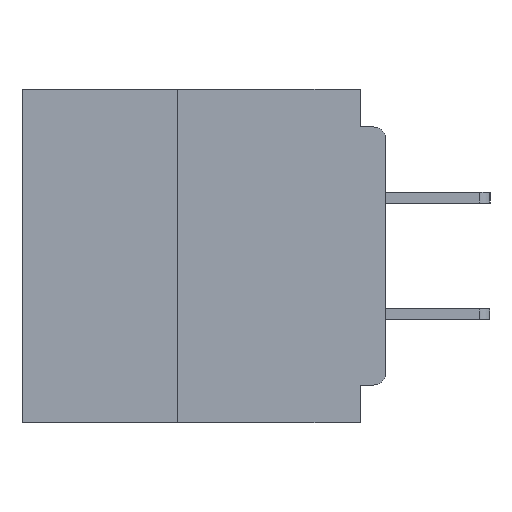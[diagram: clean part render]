
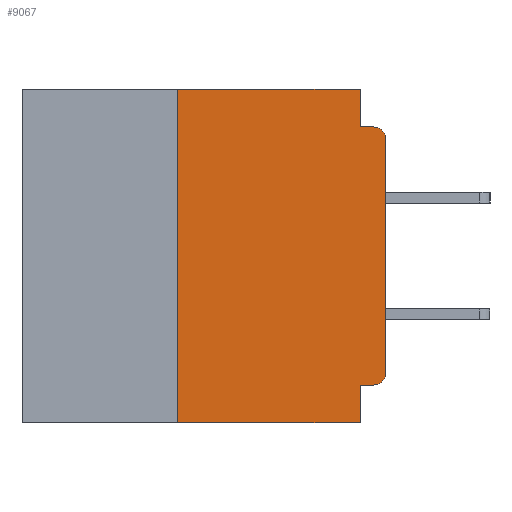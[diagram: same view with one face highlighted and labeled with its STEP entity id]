
A CAD part, left-side view. The second image highlights one B-rep face of the part: STEP entity #9067.
In plain terms, the highlighted planar face has unit normal (-1, 0, 0).
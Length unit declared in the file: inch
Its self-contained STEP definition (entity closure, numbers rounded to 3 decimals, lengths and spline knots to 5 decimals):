
#105 = CIRCLE ( 'NONE', #36105, 0.015 ) ;
#125 = ORIENTED_EDGE ( 'NONE', *, *, #11228, .F. ) ;
#563 = ORIENTED_EDGE ( 'NONE', *, *, #21620, .F. ) ;
#750 = DIRECTION ( 'NONE',  ( 0., 0., 1. ) ) ;
#1239 = CARTESIAN_POINT ( 'NONE',  ( 0., 0.031, -0.4 ) ) ;
#1869 = DIRECTION ( 'NONE',  ( 0., 1., 0. ) ) ;
#3515 = DIRECTION ( 'NONE',  ( 0., 0., -1. ) ) ;
#4103 = EDGE_LOOP ( 'NONE', ( #13863, #13553, #14789, #563, #125, #31696, #28280, #12062, #9687, #27639 ) ) ;
#4667 = CARTESIAN_POINT ( 'NONE',  ( 0., 0.031, 0. ) ) ;
#5023 = EDGE_CURVE ( 'NONE', #28924, #10430, #46100, .T. ) ;
#5041 = VERTEX_POINT ( 'NONE', #47145 ) ;
#5115 = CARTESIAN_POINT ( 'NONE',  ( 0., 0., -0.045 ) ) ;
#5302 = CARTESIAN_POINT ( 'NONE',  ( 0., 0.031, 0. ) ) ;
#5616 = LINE ( 'NONE', #36200, #42425 ) ;
#5753 = PLANE ( 'NONE',  #44428 ) ;
#6088 = VERTEX_POINT ( 'NONE', #42283 ) ;
#6740 = VECTOR ( 'NONE', #1869, 39.37008 ) ;
#6864 = EDGE_CURVE ( 'NONE', #41662, #24898, #14337, .T. ) ;
#8926 = EDGE_CURVE ( 'NONE', #46734, #6088, #25971, .T. ) ;
#9067 = ADVANCED_FACE ( 'NONE', ( #39708 ), #5753, .F. ) ;
#9687 = ORIENTED_EDGE ( 'NONE', *, *, #43727, .F. ) ;
#9796 = DIRECTION ( 'NONE',  ( -1., 0., 0. ) ) ;
#10430 = VERTEX_POINT ( 'NONE', #42661 ) ;
#10897 = CIRCLE ( 'NONE', #10925, 0.015 ) ;
#10925 = AXIS2_PLACEMENT_3D ( 'NONE', #47490, #25599, #3515 ) ;
#11228 = EDGE_CURVE ( 'NONE', #24898, #43051, #5616, .T. ) ;
#12062 = ORIENTED_EDGE ( 'NONE', *, *, #5023, .F. ) ;
#12547 = DIRECTION ( 'NONE',  ( 0., -1., 0. ) ) ;
#13178 = CARTESIAN_POINT ( 'NONE',  ( 0., 0.437, 0. ) ) ;
#13553 = ORIENTED_EDGE ( 'NONE', *, *, #17306, .T. ) ;
#13863 = ORIENTED_EDGE ( 'NONE', *, *, #33648, .T. ) ;
#14337 = LINE ( 'NONE', #16365, #32766 ) ;
#14789 = ORIENTED_EDGE ( 'NONE', *, *, #8926, .F. ) ;
#16158 = VECTOR ( 'NONE', #12547, 39.37008 ) ;
#16365 = CARTESIAN_POINT ( 'NONE',  ( 0., 0.25, -0.4 ) ) ;
#16842 = VECTOR ( 'NONE', #39131, 39.37008 ) ;
#17051 = DIRECTION ( 'NONE',  ( 0., 0., 1. ) ) ;
#17306 = EDGE_CURVE ( 'NONE', #38258, #6088, #105, .T. ) ;
#17694 = LINE ( 'NONE', #27653, #6740 ) ;
#17838 = DIRECTION ( 'NONE',  ( 0., -1., 0. ) ) ;
#20596 = DIRECTION ( 'NONE',  ( 1., 0., 0. ) ) ;
#21620 = EDGE_CURVE ( 'NONE', #43051, #46734, #24246, .T. ) ;
#21871 = LINE ( 'NONE', #43495, #41409 ) ;
#22121 = LINE ( 'NONE', #30200, #40483 ) ;
#22602 = CARTESIAN_POINT ( 'NONE',  ( 0., 0.25, -0.4 ) ) ;
#22712 = CARTESIAN_POINT ( 'NONE',  ( 0., 0.25, 0. ) ) ;
#24246 = LINE ( 'NONE', #4667, #32825 ) ;
#24295 = CARTESIAN_POINT ( 'NONE',  ( 0., 0.031, -0.045 ) ) ;
#24898 = VERTEX_POINT ( 'NONE', #22712 ) ;
#25599 = DIRECTION ( 'NONE',  ( -1., 0., 0. ) ) ;
#25788 = CARTESIAN_POINT ( 'NONE',  ( 0., 0.015, -0.355 ) ) ;
#25971 = LINE ( 'NONE', #5115, #16158 ) ;
#26922 = DIRECTION ( 'NONE',  ( 0., 0., -1. ) ) ;
#27639 = ORIENTED_EDGE ( 'NONE', *, *, #46314, .T. ) ;
#27653 = CARTESIAN_POINT ( 'NONE',  ( 0., 0., -0.355 ) ) ;
#28280 = ORIENTED_EDGE ( 'NONE', *, *, #46249, .T. ) ;
#28924 = VERTEX_POINT ( 'NONE', #35956 ) ;
#30200 = CARTESIAN_POINT ( 'NONE',  ( 0., 0., 0. ) ) ;
#30427 = CARTESIAN_POINT ( 'NONE',  ( 0., 0., -0.06 ) ) ;
#31696 = ORIENTED_EDGE ( 'NONE', *, *, #6864, .F. ) ;
#31849 = CARTESIAN_POINT ( 'NONE',  ( 0., 0.015, -0.06 ) ) ;
#32766 = VECTOR ( 'NONE', #17051, 39.37008 ) ;
#32825 = VECTOR ( 'NONE', #26922, 39.37008 ) ;
#33648 = EDGE_CURVE ( 'NONE', #5041, #38258, #22121, .T. ) ;
#35552 = DIRECTION ( 'NONE',  ( 0., 0., -1. ) ) ;
#35956 = CARTESIAN_POINT ( 'NONE',  ( 0., 0.031, -0.355 ) ) ;
#36105 = AXIS2_PLACEMENT_3D ( 'NONE', #31849, #9796, #35552 ) ;
#36200 = CARTESIAN_POINT ( 'NONE',  ( 0., 0.437, 0. ) ) ;
#38258 = VERTEX_POINT ( 'NONE', #30427 ) ;
#39131 = DIRECTION ( 'NONE',  ( 0., 0., -1. ) ) ;
#39708 = FACE_OUTER_BOUND ( 'NONE', #4103, .T. ) ;
#39812 = VERTEX_POINT ( 'NONE', #25788 ) ;
#39869 = DIRECTION ( 'NONE',  ( 0., -1., 0. ) ) ;
#40483 = VECTOR ( 'NONE', #750, 39.37008 ) ;
#41409 = VECTOR ( 'NONE', #17838, 39.37008 ) ;
#41662 = VERTEX_POINT ( 'NONE', #22602 ) ;
#42283 = CARTESIAN_POINT ( 'NONE',  ( 0., 0.015, -0.045 ) ) ;
#42425 = VECTOR ( 'NONE', #39869, 39.37008 ) ;
#42661 = CARTESIAN_POINT ( 'NONE',  ( 0., 0.031, -0.4 ) ) ;
#43051 = VERTEX_POINT ( 'NONE', #5302 ) ;
#43495 = CARTESIAN_POINT ( 'NONE',  ( 0., 0.437, -0.4 ) ) ;
#43727 = EDGE_CURVE ( 'NONE', #39812, #28924, #17694, .T. ) ;
#44428 = AXIS2_PLACEMENT_3D ( 'NONE', #13178, #20596, #46202 ) ;
#46100 = LINE ( 'NONE', #1239, #16842 ) ;
#46202 = DIRECTION ( 'NONE',  ( 0., 0., -1. ) ) ;
#46249 = EDGE_CURVE ( 'NONE', #41662, #10430, #21871, .T. ) ;
#46314 = EDGE_CURVE ( 'NONE', #39812, #5041, #10897, .T. ) ;
#46734 = VERTEX_POINT ( 'NONE', #24295 ) ;
#47145 = CARTESIAN_POINT ( 'NONE',  ( 0., 0., -0.34 ) ) ;
#47490 = CARTESIAN_POINT ( 'NONE',  ( 0., 0.015, -0.34 ) ) ;
